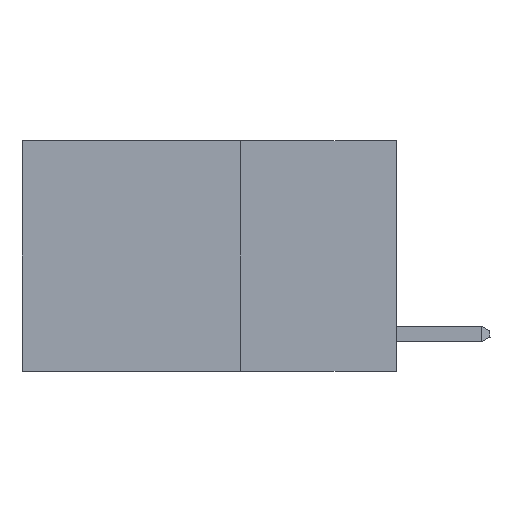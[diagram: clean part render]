
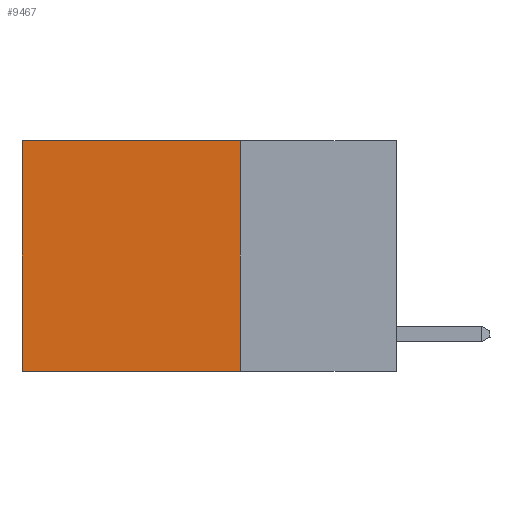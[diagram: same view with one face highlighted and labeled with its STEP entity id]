
A CAD part, left-side view. The second image highlights one B-rep face of the part: STEP entity #9467.
In plain terms, the highlighted planar face has unit normal (-1, 0, 0).
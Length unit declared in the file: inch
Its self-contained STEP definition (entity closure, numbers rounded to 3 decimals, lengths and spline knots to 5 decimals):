
#100 = CARTESIAN_POINT ( 'NONE',  ( 0.2625, 0.6, -0.37 ) ) ;
#283 = CARTESIAN_POINT ( 'NONE',  ( 0.2625, 0.25, 0. ) ) ;
#514 = CARTESIAN_POINT ( 'NONE',  ( 0.2625, 0.25, 0. ) ) ;
#2054 = DIRECTION ( 'NONE',  ( 0., 0., -1. ) ) ;
#2183 = DIRECTION ( 'NONE',  ( 1., 0., 0. ) ) ;
#2426 = AXIS2_PLACEMENT_3D ( 'NONE', #283, #2183, #2054 ) ;
#3525 = CARTESIAN_POINT ( 'NONE',  ( 0.2625, 0.25, -0.37 ) ) ;
#4349 = LINE ( 'NONE', #12066, #11180 ) ;
#4359 = EDGE_CURVE ( 'NONE', #24278, #22768, #7947, .T. ) ;
#5251 = ORIENTED_EDGE ( 'NONE', *, *, #19704, .T. ) ;
#5363 = VECTOR ( 'NONE', #14812, 39.37008 ) ;
#5931 = DIRECTION ( 'NONE',  ( 0., 1., 0. ) ) ;
#6125 = FACE_OUTER_BOUND ( 'NONE', #11553, .T. ) ;
#7775 = VERTEX_POINT ( 'NONE', #17552 ) ;
#7947 = LINE ( 'NONE', #15537, #22804 ) ;
#9467 = ADVANCED_FACE ( 'NONE', ( #6125 ), #13853, .F. ) ;
#10602 = ORIENTED_EDGE ( 'NONE', *, *, #4359, .F. ) ;
#11180 = VECTOR ( 'NONE', #19789, 39.37008 ) ;
#11553 = EDGE_LOOP ( 'NONE', ( #5251, #10602, #15483, #24620 ) ) ;
#11939 = CARTESIAN_POINT ( 'NONE',  ( 0.2625, 0.25, 0. ) ) ;
#11940 = LINE ( 'NONE', #514, #17509 ) ;
#12066 = CARTESIAN_POINT ( 'NONE',  ( 0.2625, 0.25, 0. ) ) ;
#13853 = PLANE ( 'NONE',  #2426 ) ;
#14812 = DIRECTION ( 'NONE',  ( 0., 0., -1. ) ) ;
#15483 = ORIENTED_EDGE ( 'NONE', *, *, #24827, .F. ) ;
#15537 = CARTESIAN_POINT ( 'NONE',  ( 0.2625, 0.25, -0.37 ) ) ;
#17509 = VECTOR ( 'NONE', #19913, 39.37008 ) ;
#17552 = CARTESIAN_POINT ( 'NONE',  ( 0.2625, 0.6, 0. ) ) ;
#19598 = EDGE_CURVE ( 'NONE', #24795, #7775, #11940, .T. ) ;
#19704 = EDGE_CURVE ( 'NONE', #7775, #22768, #22179, .T. ) ;
#19789 = DIRECTION ( 'NONE',  ( 0., 0., -1. ) ) ;
#19913 = DIRECTION ( 'NONE',  ( 0., 1., 0. ) ) ;
#20150 = CARTESIAN_POINT ( 'NONE',  ( 0.2625, 0.6, 0. ) ) ;
#22179 = LINE ( 'NONE', #20150, #5363 ) ;
#22768 = VERTEX_POINT ( 'NONE', #100 ) ;
#22804 = VECTOR ( 'NONE', #5931, 39.37008 ) ;
#24278 = VERTEX_POINT ( 'NONE', #3525 ) ;
#24620 = ORIENTED_EDGE ( 'NONE', *, *, #19598, .T. ) ;
#24795 = VERTEX_POINT ( 'NONE', #11939 ) ;
#24827 = EDGE_CURVE ( 'NONE', #24795, #24278, #4349, .T. ) ;
